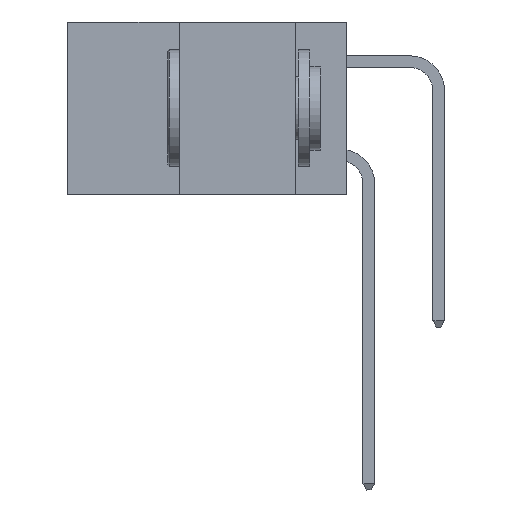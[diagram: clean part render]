
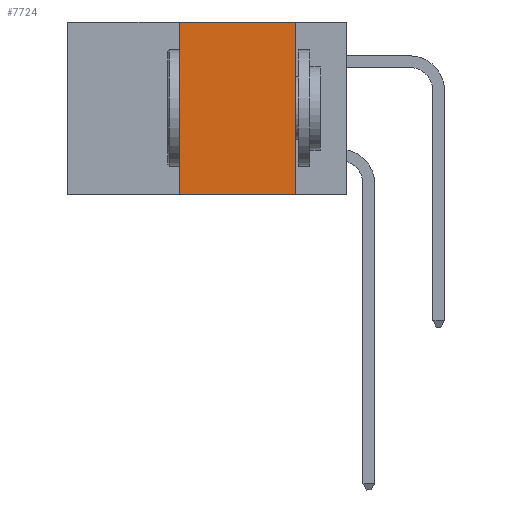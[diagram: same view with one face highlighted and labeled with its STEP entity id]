
A CAD part, left-side view. The second image highlights one B-rep face of the part: STEP entity #7724.
In plain terms, the highlighted planar face has unit normal (-1, 0, 0).
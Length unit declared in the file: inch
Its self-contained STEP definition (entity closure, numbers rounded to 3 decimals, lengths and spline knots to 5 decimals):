
#425 = LINE ( 'NONE', #16713, #19765 ) ;
#780 = CARTESIAN_POINT ( 'NONE',  ( 0., 0.11, 0. ) ) ;
#1114 = ORIENTED_EDGE ( 'NONE', *, *, #9732, .F. ) ;
#2349 = VERTEX_POINT ( 'NONE', #22994 ) ;
#2691 = EDGE_CURVE ( 'NONE', #23758, #6094, #8977, .T. ) ;
#3176 = AXIS2_PLACEMENT_3D ( 'NONE', #21343, #4539, #17697 ) ;
#3281 = CARTESIAN_POINT ( 'NONE',  ( 0., 0.36, 0. ) ) ;
#3994 = VERTEX_POINT ( 'NONE', #19654 ) ;
#4250 = VECTOR ( 'NONE', #10105, 39.37008 ) ;
#4539 = DIRECTION ( 'NONE',  ( 1., 0., 0. ) ) ;
#5691 = CARTESIAN_POINT ( 'NONE',  ( 0., 0.36, -0.37 ) ) ;
#5869 = LINE ( 'NONE', #3281, #9137 ) ;
#6094 = VERTEX_POINT ( 'NONE', #24195 ) ;
#7724 = ADVANCED_FACE ( 'NONE', ( #19587 ), #15799, .F. ) ;
#8977 = LINE ( 'NONE', #17486, #18933 ) ;
#9137 = VECTOR ( 'NONE', #14545, 39.37008 ) ;
#9223 = DIRECTION ( 'NONE',  ( 0., -1., 0. ) ) ;
#9732 = EDGE_CURVE ( 'NONE', #3994, #6094, #24163, .T. ) ;
#10105 = DIRECTION ( 'NONE',  ( 0., 0., -1. ) ) ;
#11964 = EDGE_CURVE ( 'NONE', #23758, #2349, #5869, .T. ) ;
#14545 = DIRECTION ( 'NONE',  ( 0., 0., 1. ) ) ;
#14980 = ORIENTED_EDGE ( 'NONE', *, *, #11964, .F. ) ;
#14982 = ORIENTED_EDGE ( 'NONE', *, *, #2691, .T. ) ;
#15799 = PLANE ( 'NONE',  #3176 ) ;
#16713 = CARTESIAN_POINT ( 'NONE',  ( 0., 0.6, 0. ) ) ;
#17449 = DIRECTION ( 'NONE',  ( 0., -1., 0. ) ) ;
#17486 = CARTESIAN_POINT ( 'NONE',  ( 0., 0.6, -0.37 ) ) ;
#17697 = DIRECTION ( 'NONE',  ( 0., 0., -1. ) ) ;
#18933 = VECTOR ( 'NONE', #17449, 39.37008 ) ;
#19137 = EDGE_CURVE ( 'NONE', #2349, #3994, #425, .T. ) ;
#19587 = FACE_OUTER_BOUND ( 'NONE', #23656, .T. ) ;
#19654 = CARTESIAN_POINT ( 'NONE',  ( 0., 0.11, 0. ) ) ;
#19765 = VECTOR ( 'NONE', #9223, 39.37008 ) ;
#21311 = ORIENTED_EDGE ( 'NONE', *, *, #19137, .F. ) ;
#21343 = CARTESIAN_POINT ( 'NONE',  ( 0., 0.6, 0. ) ) ;
#22994 = CARTESIAN_POINT ( 'NONE',  ( 0., 0.36, 0. ) ) ;
#23656 = EDGE_LOOP ( 'NONE', ( #1114, #21311, #14980, #14982 ) ) ;
#23758 = VERTEX_POINT ( 'NONE', #5691 ) ;
#24163 = LINE ( 'NONE', #780, #4250 ) ;
#24195 = CARTESIAN_POINT ( 'NONE',  ( 0., 0.11, -0.37 ) ) ;
